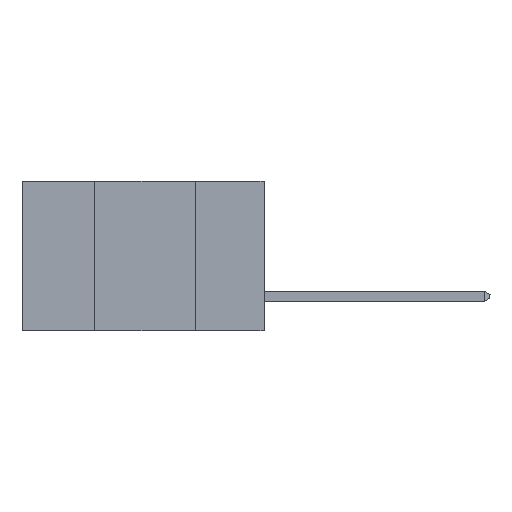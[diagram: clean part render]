
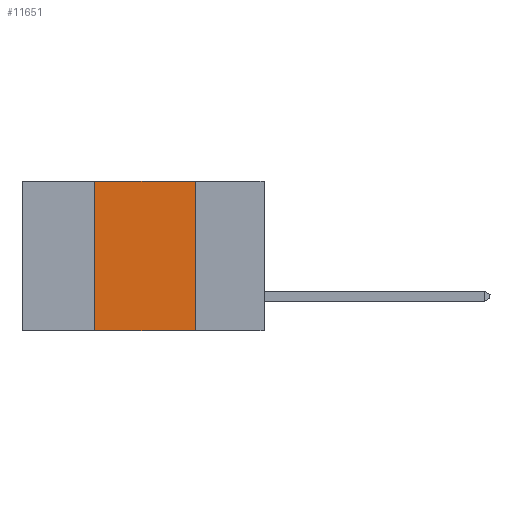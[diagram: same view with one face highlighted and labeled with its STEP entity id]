
A CAD part, left-side view. The second image highlights one B-rep face of the part: STEP entity #11651.
In plain terms, the highlighted planar face has unit normal (-1, 0, 0).
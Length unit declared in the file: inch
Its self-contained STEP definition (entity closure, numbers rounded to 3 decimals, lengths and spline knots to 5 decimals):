
#209 = VERTEX_POINT ( 'NONE', #14695 ) ;
#579 = CARTESIAN_POINT ( 'NONE',  ( 0., 0.17, -0.37 ) ) ;
#672 = ORIENTED_EDGE ( 'NONE', *, *, #3832, .T. ) ;
#990 = CARTESIAN_POINT ( 'NONE',  ( 0., 0.42, -0.37 ) ) ;
#1256 = LINE ( 'NONE', #2661, #15903 ) ;
#1264 = VECTOR ( 'NONE', #17029, 39.37008 ) ;
#1451 = VECTOR ( 'NONE', #3311, 39.37008 ) ;
#2486 = CARTESIAN_POINT ( 'NONE',  ( 0., 0.6, 0. ) ) ;
#2652 = EDGE_CURVE ( 'NONE', #3280, #14198, #11660, .T. ) ;
#2661 = CARTESIAN_POINT ( 'NONE',  ( 0., 0.6, -0.37 ) ) ;
#3153 = CARTESIAN_POINT ( 'NONE',  ( 0., 0.42, -0.37 ) ) ;
#3280 = VERTEX_POINT ( 'NONE', #3153 ) ;
#3311 = DIRECTION ( 'NONE',  ( 0., 0., -1. ) ) ;
#3379 = EDGE_LOOP ( 'NONE', ( #5465, #8635, #3544, #672 ) ) ;
#3544 = ORIENTED_EDGE ( 'NONE', *, *, #2652, .F. ) ;
#3832 = EDGE_CURVE ( 'NONE', #3280, #209, #1256, .T. ) ;
#3848 = DIRECTION ( 'NONE',  ( 0., 0., -1. ) ) ;
#3899 = EDGE_CURVE ( 'NONE', #14198, #8630, #14578, .T. ) ;
#5465 = ORIENTED_EDGE ( 'NONE', *, *, #13626, .F. ) ;
#6307 = PLANE ( 'NONE',  #14694 ) ;
#7217 = VECTOR ( 'NONE', #9183, 39.37008 ) ;
#7241 = CARTESIAN_POINT ( 'NONE',  ( 0., 0.17, 0. ) ) ;
#8630 = VERTEX_POINT ( 'NONE', #7241 ) ;
#8635 = ORIENTED_EDGE ( 'NONE', *, *, #3899, .F. ) ;
#9183 = DIRECTION ( 'NONE',  ( 0., 0., 1. ) ) ;
#11651 = ADVANCED_FACE ( 'NONE', ( #16962 ), #6307, .F. ) ;
#11660 = LINE ( 'NONE', #990, #7217 ) ;
#13626 = EDGE_CURVE ( 'NONE', #8630, #209, #13808, .T. ) ;
#13808 = LINE ( 'NONE', #579, #1451 ) ;
#14198 = VERTEX_POINT ( 'NONE', #15957 ) ;
#14578 = LINE ( 'NONE', #2486, #1264 ) ;
#14694 = AXIS2_PLACEMENT_3D ( 'NONE', #15914, #15566, #3848 ) ;
#14695 = CARTESIAN_POINT ( 'NONE',  ( 0., 0.17, -0.37 ) ) ;
#14747 = DIRECTION ( 'NONE',  ( 0., -1., 0. ) ) ;
#15566 = DIRECTION ( 'NONE',  ( 1., 0., 0. ) ) ;
#15903 = VECTOR ( 'NONE', #14747, 39.37008 ) ;
#15914 = CARTESIAN_POINT ( 'NONE',  ( 0., 0.6, 0. ) ) ;
#15957 = CARTESIAN_POINT ( 'NONE',  ( 0., 0.42, 0. ) ) ;
#16962 = FACE_OUTER_BOUND ( 'NONE', #3379, .T. ) ;
#17029 = DIRECTION ( 'NONE',  ( 0., -1., 0. ) ) ;
